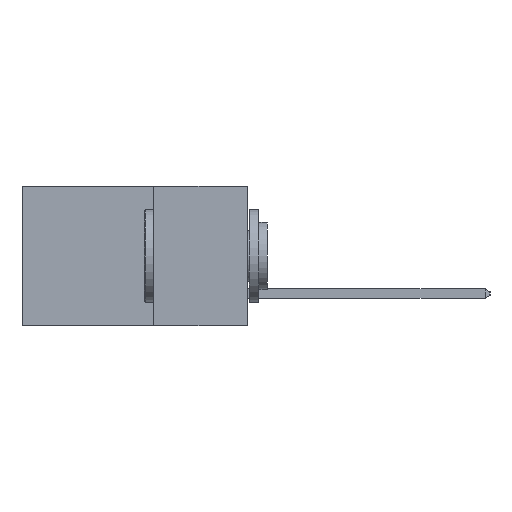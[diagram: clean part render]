
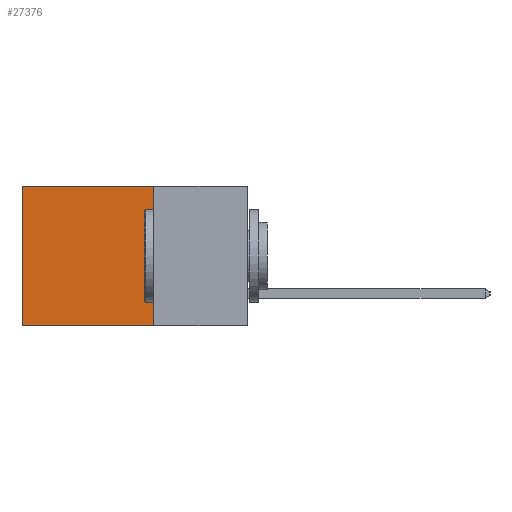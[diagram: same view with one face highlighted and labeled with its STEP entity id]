
A CAD part, left-side view. The second image highlights one B-rep face of the part: STEP entity #27376.
In plain terms, the highlighted planar face has unit normal (-1, 0, 0).
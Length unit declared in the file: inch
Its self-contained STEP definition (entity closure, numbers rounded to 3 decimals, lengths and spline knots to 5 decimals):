
#406 = CARTESIAN_POINT ( 'NONE',  ( 0.298, 0.6, 0. ) ) ;
#509 = DIRECTION ( 'NONE',  ( 0., 0., -1. ) ) ;
#762 = CARTESIAN_POINT ( 'NONE',  ( 0.298, 0.25, -0.37 ) ) ;
#1009 = CARTESIAN_POINT ( 'NONE',  ( 0.298, 0.25, 0. ) ) ;
#3246 = LINE ( 'NONE', #1009, #8973 ) ;
#3580 = LINE ( 'NONE', #762, #29030 ) ;
#4036 = VERTEX_POINT ( 'NONE', #9946 ) ;
#6119 = ORIENTED_EDGE ( 'NONE', *, *, #7026, .T. ) ;
#6442 = VERTEX_POINT ( 'NONE', #8558 ) ;
#6730 = ORIENTED_EDGE ( 'NONE', *, *, #10937, .T. ) ;
#7026 = EDGE_CURVE ( 'NONE', #16632, #4036, #20635, .T. ) ;
#7451 = VECTOR ( 'NONE', #509, 39.37008 ) ;
#7743 = EDGE_LOOP ( 'NONE', ( #6119, #17970, #24189, #6730 ) ) ;
#8224 = VECTOR ( 'NONE', #14400, 39.37008 ) ;
#8558 = CARTESIAN_POINT ( 'NONE',  ( 0.298, 0.25, 0. ) ) ;
#8973 = VECTOR ( 'NONE', #15772, 39.37008 ) ;
#9405 = CARTESIAN_POINT ( 'NONE',  ( 0.298, 0.25, 0. ) ) ;
#9795 = CARTESIAN_POINT ( 'NONE',  ( 0.298, 0.25, 0. ) ) ;
#9946 = CARTESIAN_POINT ( 'NONE',  ( 0.298, 0.6, -0.37 ) ) ;
#10937 = EDGE_CURVE ( 'NONE', #6442, #16632, #3246, .T. ) ;
#11558 = EDGE_CURVE ( 'NONE', #31151, #4036, #3580, .T. ) ;
#12293 = DIRECTION ( 'NONE',  ( 0., 0., -1. ) ) ;
#14400 = DIRECTION ( 'NONE',  ( 0., 0., -1. ) ) ;
#14913 = FACE_OUTER_BOUND ( 'NONE', #7743, .T. ) ;
#15772 = DIRECTION ( 'NONE',  ( 0., 1., 0. ) ) ;
#16632 = VERTEX_POINT ( 'NONE', #29063 ) ;
#17970 = ORIENTED_EDGE ( 'NONE', *, *, #11558, .F. ) ;
#18026 = DIRECTION ( 'NONE',  ( 0., 1., 0. ) ) ;
#18683 = EDGE_CURVE ( 'NONE', #6442, #31151, #21420, .T. ) ;
#19493 = AXIS2_PLACEMENT_3D ( 'NONE', #9795, #27120, #12293 ) ;
#20635 = LINE ( 'NONE', #406, #7451 ) ;
#21420 = LINE ( 'NONE', #9405, #8224 ) ;
#24189 = ORIENTED_EDGE ( 'NONE', *, *, #18683, .F. ) ;
#27109 = CARTESIAN_POINT ( 'NONE',  ( 0.298, 0.25, -0.37 ) ) ;
#27120 = DIRECTION ( 'NONE',  ( 1., 0., 0. ) ) ;
#27376 = ADVANCED_FACE ( 'NONE', ( #14913 ), #29332, .F. ) ;
#29030 = VECTOR ( 'NONE', #18026, 39.37008 ) ;
#29063 = CARTESIAN_POINT ( 'NONE',  ( 0.298, 0.6, 0. ) ) ;
#29332 = PLANE ( 'NONE',  #19493 ) ;
#31151 = VERTEX_POINT ( 'NONE', #27109 ) ;
